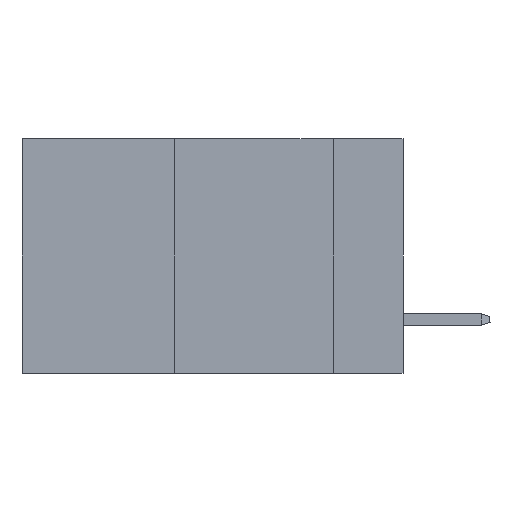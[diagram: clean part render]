
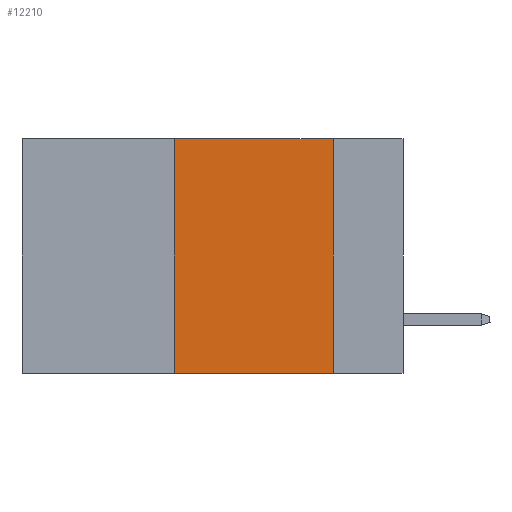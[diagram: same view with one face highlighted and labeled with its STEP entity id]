
A CAD part, left-side view. The second image highlights one B-rep face of the part: STEP entity #12210.
In plain terms, the highlighted planar face has unit normal (-1, 0, 0).
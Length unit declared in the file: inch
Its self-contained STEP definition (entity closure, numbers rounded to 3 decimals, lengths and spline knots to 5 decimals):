
#585 = EDGE_CURVE ( 'NONE', #6560, #9170, #2873, .T. ) ;
#1326 = FACE_OUTER_BOUND ( 'NONE', #7515, .T. ) ;
#2208 = LINE ( 'NONE', #29820, #31727 ) ;
#2372 = VERTEX_POINT ( 'NONE', #28647 ) ;
#2873 = LINE ( 'NONE', #13097, #4061 ) ;
#3503 = ORIENTED_EDGE ( 'NONE', *, *, #11145, .F. ) ;
#4061 = VECTOR ( 'NONE', #8626, 39.37008 ) ;
#6560 = VERTEX_POINT ( 'NONE', #18596 ) ;
#7515 = EDGE_LOOP ( 'NONE', ( #16110, #8362, #3503, #23568 ) ) ;
#8048 = CARTESIAN_POINT ( 'NONE',  ( 0., 0.11, 0. ) ) ;
#8362 = ORIENTED_EDGE ( 'NONE', *, *, #19785, .F. ) ;
#8626 = DIRECTION ( 'NONE',  ( 0., -1., 0. ) ) ;
#9170 = VERTEX_POINT ( 'NONE', #21871 ) ;
#9986 = DIRECTION ( 'NONE',  ( 0., 0., 1. ) ) ;
#11145 = EDGE_CURVE ( 'NONE', #6560, #2372, #14441, .T. ) ;
#12210 = ADVANCED_FACE ( 'NONE', ( #1326 ), #20896, .F. ) ;
#13097 = CARTESIAN_POINT ( 'NONE',  ( 0., 0.6, -0.37 ) ) ;
#14441 = LINE ( 'NONE', #31996, #21522 ) ;
#14832 = EDGE_CURVE ( 'NONE', #16420, #9170, #21434, .T. ) ;
#15804 = CARTESIAN_POINT ( 'NONE',  ( 0., 0.6, 0. ) ) ;
#16110 = ORIENTED_EDGE ( 'NONE', *, *, #14832, .F. ) ;
#16134 = DIRECTION ( 'NONE',  ( 0., 0., -1. ) ) ;
#16420 = VERTEX_POINT ( 'NONE', #8048 ) ;
#18596 = CARTESIAN_POINT ( 'NONE',  ( 0., 0.36, -0.37 ) ) ;
#18919 = DIRECTION ( 'NONE',  ( 1., 0., 0. ) ) ;
#19785 = EDGE_CURVE ( 'NONE', #2372, #16420, #2208, .T. ) ;
#20896 = PLANE ( 'NONE',  #31561 ) ;
#21434 = LINE ( 'NONE', #31268, #25311 ) ;
#21522 = VECTOR ( 'NONE', #9986, 39.37008 ) ;
#21871 = CARTESIAN_POINT ( 'NONE',  ( 0., 0.11, -0.37 ) ) ;
#22578 = DIRECTION ( 'NONE',  ( 0., -1., 0. ) ) ;
#23568 = ORIENTED_EDGE ( 'NONE', *, *, #585, .T. ) ;
#24380 = DIRECTION ( 'NONE',  ( 0., 0., -1. ) ) ;
#25311 = VECTOR ( 'NONE', #24380, 39.37008 ) ;
#28647 = CARTESIAN_POINT ( 'NONE',  ( 0., 0.36, 0. ) ) ;
#29820 = CARTESIAN_POINT ( 'NONE',  ( 0., 0.6, 0. ) ) ;
#31268 = CARTESIAN_POINT ( 'NONE',  ( 0., 0.11, 0. ) ) ;
#31561 = AXIS2_PLACEMENT_3D ( 'NONE', #15804, #18919, #16134 ) ;
#31727 = VECTOR ( 'NONE', #22578, 39.37008 ) ;
#31996 = CARTESIAN_POINT ( 'NONE',  ( 0., 0.36, 0. ) ) ;
